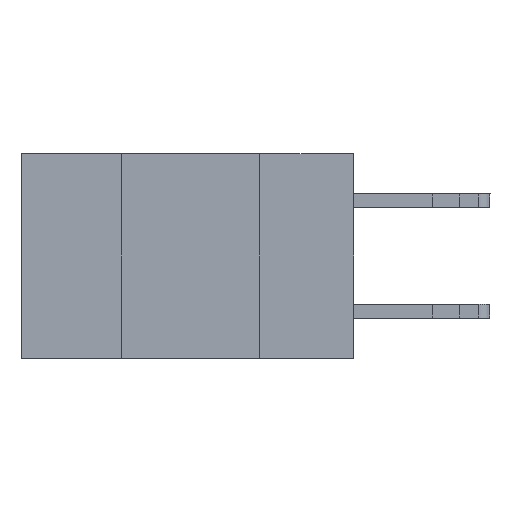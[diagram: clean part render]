
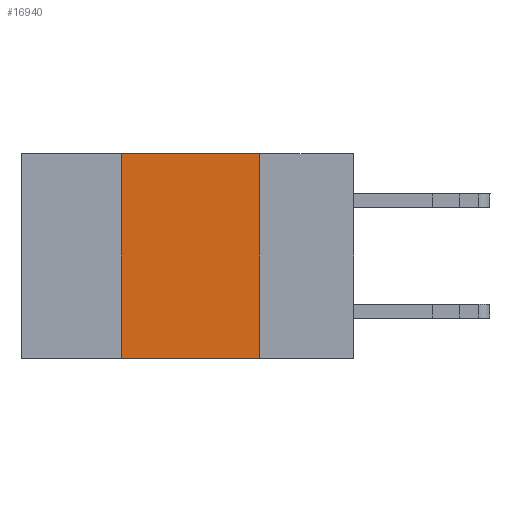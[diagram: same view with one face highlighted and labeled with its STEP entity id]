
A CAD part, left-side view. The second image highlights one B-rep face of the part: STEP entity #16940.
In plain terms, the highlighted planar face has unit normal (-1, 0, 0).
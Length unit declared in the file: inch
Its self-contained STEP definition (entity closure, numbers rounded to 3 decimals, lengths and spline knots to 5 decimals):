
#415 = VERTEX_POINT ( 'NONE', #33517 ) ;
#1261 = EDGE_CURVE ( 'NONE', #415, #22884, #17775, .T. ) ;
#3067 = LINE ( 'NONE', #15234, #35208 ) ;
#3231 = VECTOR ( 'NONE', #12089, 39.37008 ) ;
#3686 = CARTESIAN_POINT ( 'NONE',  ( 0., 0.6, -0.37 ) ) ;
#6238 = CARTESIAN_POINT ( 'NONE',  ( 0., 0.6, 0. ) ) ;
#7084 = ORIENTED_EDGE ( 'NONE', *, *, #25972, .F. ) ;
#8021 = CARTESIAN_POINT ( 'NONE',  ( 0., 0.17, 0. ) ) ;
#8358 = LINE ( 'NONE', #8021, #25054 ) ;
#8985 = DIRECTION ( 'NONE',  ( 0., 0., -1. ) ) ;
#9758 = DIRECTION ( 'NONE',  ( 0., 0., 1. ) ) ;
#9897 = LINE ( 'NONE', #22939, #28763 ) ;
#11581 = VERTEX_POINT ( 'NONE', #23006 ) ;
#12089 = DIRECTION ( 'NONE',  ( 0., -1., 0. ) ) ;
#14514 = ORIENTED_EDGE ( 'NONE', *, *, #19167, .F. ) ;
#14815 = DIRECTION ( 'NONE',  ( 0., -1., 0. ) ) ;
#15234 = CARTESIAN_POINT ( 'NONE',  ( 0., 0.42, 0. ) ) ;
#15547 = CARTESIAN_POINT ( 'NONE',  ( 0., 0.17, -0.37 ) ) ;
#16940 = ADVANCED_FACE ( 'NONE', ( #30197 ), #22584, .F. ) ;
#17775 = LINE ( 'NONE', #3686, #3231 ) ;
#18060 = CARTESIAN_POINT ( 'NONE',  ( 0., 0.17, 0. ) ) ;
#18211 = ORIENTED_EDGE ( 'NONE', *, *, #1261, .T. ) ;
#18960 = DIRECTION ( 'NONE',  ( 0., 0., -1. ) ) ;
#19114 = ORIENTED_EDGE ( 'NONE', *, *, #34799, .F. ) ;
#19167 = EDGE_CURVE ( 'NONE', #22199, #22884, #8358, .T. ) ;
#22199 = VERTEX_POINT ( 'NONE', #18060 ) ;
#22584 = PLANE ( 'NONE',  #29410 ) ;
#22884 = VERTEX_POINT ( 'NONE', #15547 ) ;
#22939 = CARTESIAN_POINT ( 'NONE',  ( 0., 0.6, 0. ) ) ;
#23006 = CARTESIAN_POINT ( 'NONE',  ( 0., 0.42, 0. ) ) ;
#25054 = VECTOR ( 'NONE', #18960, 39.37008 ) ;
#25407 = DIRECTION ( 'NONE',  ( 1., 0., 0. ) ) ;
#25972 = EDGE_CURVE ( 'NONE', #11581, #22199, #9897, .T. ) ;
#28763 = VECTOR ( 'NONE', #14815, 39.37008 ) ;
#29410 = AXIS2_PLACEMENT_3D ( 'NONE', #6238, #25407, #8985 ) ;
#30197 = FACE_OUTER_BOUND ( 'NONE', #31768, .T. ) ;
#31768 = EDGE_LOOP ( 'NONE', ( #14514, #7084, #19114, #18211 ) ) ;
#33517 = CARTESIAN_POINT ( 'NONE',  ( 0., 0.42, -0.37 ) ) ;
#34799 = EDGE_CURVE ( 'NONE', #415, #11581, #3067, .T. ) ;
#35208 = VECTOR ( 'NONE', #9758, 39.37008 ) ;
